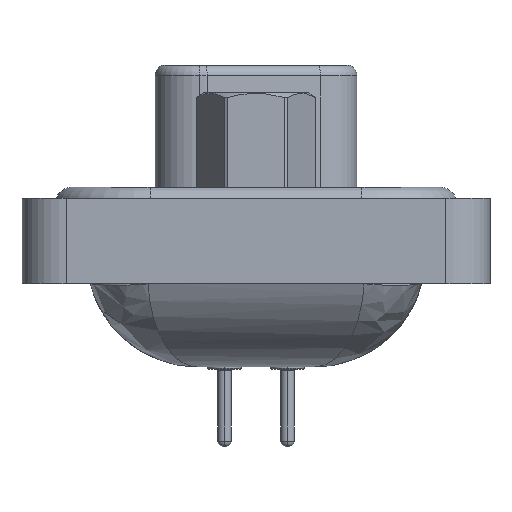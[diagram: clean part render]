
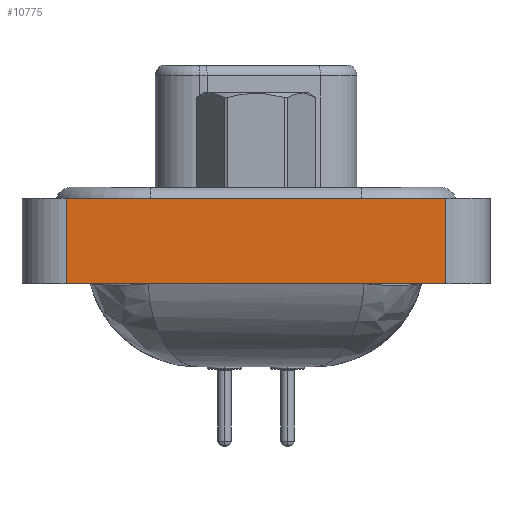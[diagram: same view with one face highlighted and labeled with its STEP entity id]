
A CAD part, left-side view. The second image highlights one B-rep face of the part: STEP entity #10775.
In plain terms, the highlighted planar face has unit normal (-1, 0, 0).
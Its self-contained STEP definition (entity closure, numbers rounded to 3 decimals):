
#183 = DIRECTION ( 'NONE',  ( 0., 0., 1. ) ) ;
#600 = VERTEX_POINT ( 'NONE', #9192 ) ;
#1401 = EDGE_CURVE ( 'NONE', #17765, #8307, #5577, .T. ) ;
#2676 = LINE ( 'NONE', #16884, #13585 ) ;
#3619 = DIRECTION ( 'NONE',  ( 0., -1., 0. ) ) ;
#3887 = EDGE_CURVE ( 'NONE', #8307, #600, #6961, .T. ) ;
#4589 = EDGE_CURVE ( 'NONE', #19691, #600, #7947, .T. ) ;
#4679 = CARTESIAN_POINT ( 'NONE',  ( -7.25, -8.55, -3.35 ) ) ;
#5325 = EDGE_CURVE ( 'NONE', #17765, #19691, #2676, .T. ) ;
#5577 = LINE ( 'NONE', #8649, #15433 ) ;
#5970 = CARTESIAN_POINT ( 'NONE',  ( -7.25, 8.55, 0.5 ) ) ;
#6441 = PLANE ( 'NONE',  #8533 ) ;
#6961 = LINE ( 'NONE', #17825, #7984 ) ;
#7947 = LINE ( 'NONE', #4679, #19446 ) ;
#7984 = VECTOR ( 'NONE', #3619, 1000. ) ;
#8307 = VERTEX_POINT ( 'NONE', #5970 ) ;
#8533 = AXIS2_PLACEMENT_3D ( 'NONE', #15658, #15854, #19026 ) ;
#8649 = CARTESIAN_POINT ( 'NONE',  ( -7.25, 8.55, -3.35 ) ) ;
#9192 = CARTESIAN_POINT ( 'NONE',  ( -7.25, -8.55, 0.5 ) ) ;
#9665 = EDGE_LOOP ( 'NONE', ( #15585, #18983, #12075, #12588 ) ) ;
#10535 = DIRECTION ( 'NONE',  ( 0., -1., 0. ) ) ;
#10775 = ADVANCED_FACE ( 'NONE', ( #12899 ), #6441, .T. ) ;
#11658 = CARTESIAN_POINT ( 'NONE',  ( -7.25, -8.55, -3.35 ) ) ;
#12075 = ORIENTED_EDGE ( 'NONE', *, *, #1401, .F. ) ;
#12588 = ORIENTED_EDGE ( 'NONE', *, *, #5325, .T. ) ;
#12899 = FACE_OUTER_BOUND ( 'NONE', #9665, .T. ) ;
#13585 = VECTOR ( 'NONE', #10535, 1000. ) ;
#15391 = CARTESIAN_POINT ( 'NONE',  ( -7.25, 8.55, -3.35 ) ) ;
#15433 = VECTOR ( 'NONE', #16532, 1000. ) ;
#15585 = ORIENTED_EDGE ( 'NONE', *, *, #4589, .T. ) ;
#15658 = CARTESIAN_POINT ( 'NONE',  ( -7.25, -8.55, -3.35 ) ) ;
#15854 = DIRECTION ( 'NONE',  ( -1., 0., 0. ) ) ;
#16532 = DIRECTION ( 'NONE',  ( 0., 0., 1. ) ) ;
#16884 = CARTESIAN_POINT ( 'NONE',  ( -7.25, -8.55, -3.35 ) ) ;
#17765 = VERTEX_POINT ( 'NONE', #15391 ) ;
#17825 = CARTESIAN_POINT ( 'NONE',  ( -7.25, -8.55, 0.5 ) ) ;
#18983 = ORIENTED_EDGE ( 'NONE', *, *, #3887, .F. ) ;
#19026 = DIRECTION ( 'NONE',  ( 0., 0., 1. ) ) ;
#19446 = VECTOR ( 'NONE', #183, 1000. ) ;
#19691 = VERTEX_POINT ( 'NONE', #11658 ) ;
